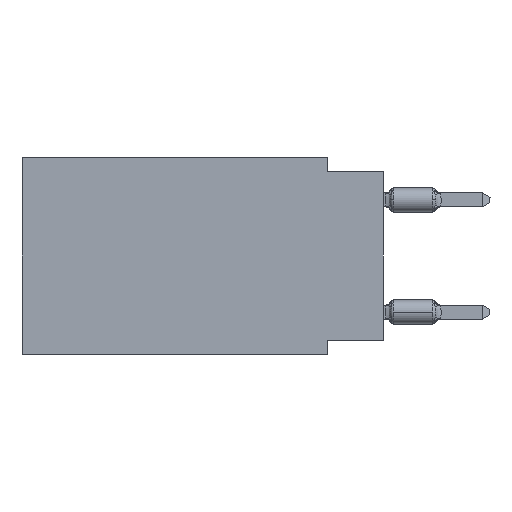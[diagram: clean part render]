
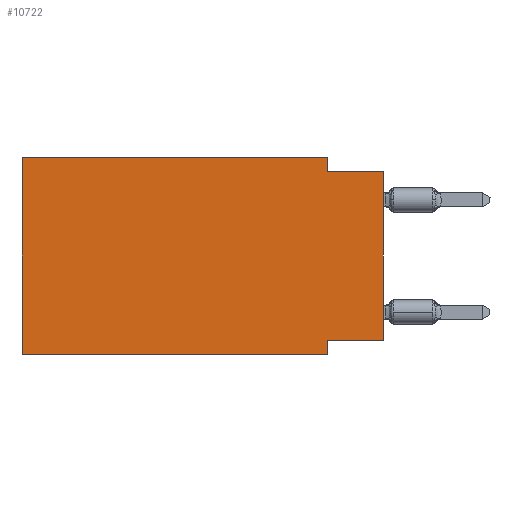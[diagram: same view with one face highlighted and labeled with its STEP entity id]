
A CAD part, left-side view. The second image highlights one B-rep face of the part: STEP entity #10722.
In plain terms, the highlighted planar face has unit normal (-1, 0, 0).
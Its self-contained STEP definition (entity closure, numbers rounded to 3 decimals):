
#1181 = DIRECTION ( 'NONE',  ( 0., 1., 0. ) ) ;
#1894 = EDGE_CURVE ( 'NONE', #42836, #10895, #38239, .T. ) ;
#1970 = CARTESIAN_POINT ( 'NONE',  ( 0., 16.383, 0. ) ) ;
#2250 = CARTESIAN_POINT ( 'NONE',  ( 0., 16.383, 0. ) ) ;
#2259 = ORIENTED_EDGE ( 'NONE', *, *, #5418, .F. ) ;
#2966 = CARTESIAN_POINT ( 'NONE',  ( 0., 16.383, -8.89 ) ) ;
#3613 = CARTESIAN_POINT ( 'NONE',  ( 0., 0., -0.635 ) ) ;
#3875 = ORIENTED_EDGE ( 'NONE', *, *, #23405, .T. ) ;
#4418 = AXIS2_PLACEMENT_3D ( 'NONE', #29764, #10029, #33222 ) ;
#5057 = DIRECTION ( 'NONE',  ( 0., 0., 1. ) ) ;
#5418 = EDGE_CURVE ( 'NONE', #16169, #33423, #38059, .T. ) ;
#5792 = DIRECTION ( 'NONE',  ( 0., -1., 0. ) ) ;
#5840 = EDGE_CURVE ( 'NONE', #9335, #25802, #24154, .T. ) ;
#6207 = LINE ( 'NONE', #2966, #34351 ) ;
#6243 = DIRECTION ( 'NONE',  ( 0., -1., 0. ) ) ;
#6430 = EDGE_CURVE ( 'NONE', #10895, #16169, #23590, .T. ) ;
#7928 = ORIENTED_EDGE ( 'NONE', *, *, #22565, .F. ) ;
#9228 = DIRECTION ( 'NONE',  ( 0., 0., -1. ) ) ;
#9335 = VERTEX_POINT ( 'NONE', #31296 ) ;
#9668 = VECTOR ( 'NONE', #9228, 1000. ) ;
#9947 = CARTESIAN_POINT ( 'NONE',  ( 0., 0., -0.635 ) ) ;
#10029 = DIRECTION ( 'NONE',  ( 1., 0., 0. ) ) ;
#10475 = EDGE_CURVE ( 'NONE', #9335, #40278, #25012, .T. ) ;
#10722 = ADVANCED_FACE ( 'NONE', ( #23910 ), #36916, .F. ) ;
#10895 = VERTEX_POINT ( 'NONE', #1970 ) ;
#11257 = ORIENTED_EDGE ( 'NONE', *, *, #10475, .T. ) ;
#11571 = EDGE_LOOP ( 'NONE', ( #11257, #35417, #2259, #38975, #36999, #3875, #7928, #13062 ) ) ;
#12232 = LINE ( 'NONE', #25464, #15101 ) ;
#12728 = VECTOR ( 'NONE', #5057, 1000. ) ;
#13062 = ORIENTED_EDGE ( 'NONE', *, *, #5840, .F. ) ;
#14216 = VECTOR ( 'NONE', #1181, 1000. ) ;
#15101 = VECTOR ( 'NONE', #38687, 1000. ) ;
#16169 = VERTEX_POINT ( 'NONE', #19670 ) ;
#17367 = VECTOR ( 'NONE', #31516, 1000. ) ;
#17508 = CARTESIAN_POINT ( 'NONE',  ( 0., 2.54, -0.635 ) ) ;
#19670 = CARTESIAN_POINT ( 'NONE',  ( 0., 2.54, 0. ) ) ;
#19708 = DIRECTION ( 'NONE',  ( 0., -1., 0. ) ) ;
#20362 = CARTESIAN_POINT ( 'NONE',  ( 0., 16.383, 0. ) ) ;
#20803 = CARTESIAN_POINT ( 'NONE',  ( 0., 16.383, -8.89 ) ) ;
#21827 = CARTESIAN_POINT ( 'NONE',  ( 0., 2.54, 0. ) ) ;
#22565 = EDGE_CURVE ( 'NONE', #25802, #29059, #12232, .T. ) ;
#23405 = EDGE_CURVE ( 'NONE', #42836, #29059, #6207, .T. ) ;
#23590 = LINE ( 'NONE', #20362, #34999 ) ;
#23910 = FACE_OUTER_BOUND ( 'NONE', #11571, .T. ) ;
#24154 = LINE ( 'NONE', #37801, #14216 ) ;
#25012 = LINE ( 'NONE', #28049, #12728 ) ;
#25424 = EDGE_CURVE ( 'NONE', #33423, #40278, #25995, .T. ) ;
#25464 = CARTESIAN_POINT ( 'NONE',  ( 0., 2.54, -8.89 ) ) ;
#25802 = VERTEX_POINT ( 'NONE', #29416 ) ;
#25995 = LINE ( 'NONE', #9947, #41783 ) ;
#28049 = CARTESIAN_POINT ( 'NONE',  ( 0., 0., 0. ) ) ;
#29059 = VERTEX_POINT ( 'NONE', #33864 ) ;
#29416 = CARTESIAN_POINT ( 'NONE',  ( 0., 2.54, -8.255 ) ) ;
#29764 = CARTESIAN_POINT ( 'NONE',  ( 0., 16.383, 0. ) ) ;
#31296 = CARTESIAN_POINT ( 'NONE',  ( 0., 0., -8.255 ) ) ;
#31516 = DIRECTION ( 'NONE',  ( 0., 0., 1. ) ) ;
#33222 = DIRECTION ( 'NONE',  ( 0., 0., -1. ) ) ;
#33423 = VERTEX_POINT ( 'NONE', #17508 ) ;
#33864 = CARTESIAN_POINT ( 'NONE',  ( 0., 2.54, -8.89 ) ) ;
#34351 = VECTOR ( 'NONE', #5792, 1000. ) ;
#34999 = VECTOR ( 'NONE', #19708, 1000. ) ;
#35417 = ORIENTED_EDGE ( 'NONE', *, *, #25424, .F. ) ;
#36916 = PLANE ( 'NONE',  #4418 ) ;
#36999 = ORIENTED_EDGE ( 'NONE', *, *, #1894, .F. ) ;
#37801 = CARTESIAN_POINT ( 'NONE',  ( 0., 0., -8.255 ) ) ;
#38059 = LINE ( 'NONE', #21827, #9668 ) ;
#38239 = LINE ( 'NONE', #2250, #17367 ) ;
#38687 = DIRECTION ( 'NONE',  ( 0., 0., -1. ) ) ;
#38975 = ORIENTED_EDGE ( 'NONE', *, *, #6430, .F. ) ;
#40278 = VERTEX_POINT ( 'NONE', #3613 ) ;
#41783 = VECTOR ( 'NONE', #6243, 1000. ) ;
#42836 = VERTEX_POINT ( 'NONE', #20803 ) ;
